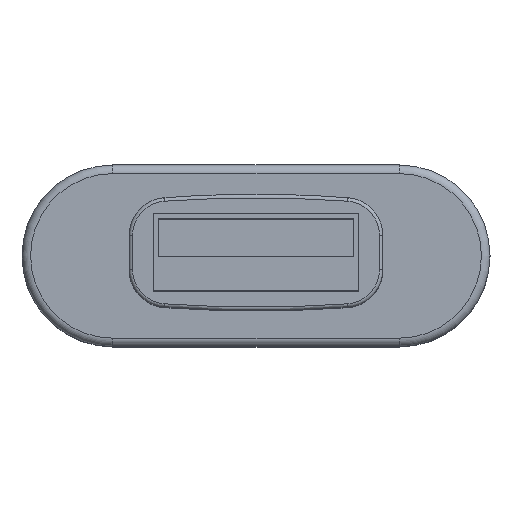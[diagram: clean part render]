
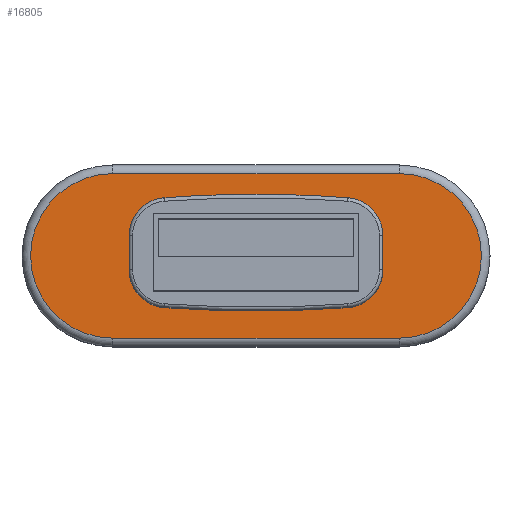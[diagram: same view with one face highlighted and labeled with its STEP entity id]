
A CAD part, top view. The second image highlights one B-rep face of the part: STEP entity #16805.
In plain terms, the highlighted planar face has unit normal (0, 0, 1).
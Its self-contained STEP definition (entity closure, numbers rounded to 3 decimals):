
#1 = EDGE_CURVE ( 'NONE', #7623, #8431, #138, .T. ) ;
#138 = LINE ( 'NONE', #15541, #14662 ) ;
#560 = CARTESIAN_POINT ( 'NONE',  ( -2.75, 0., 11.9 ) ) ;
#772 = CARTESIAN_POINT ( 'NONE',  ( 0., 0., 11.9 ) ) ;
#1634 = ORIENTED_EDGE ( 'NONE', *, *, #1, .T. ) ;
#2061 = AXIS2_PLACEMENT_3D ( 'NONE', #13892, #9554, #3925 ) ;
#2501 = EDGE_CURVE ( 'NONE', #7623, #11617, #17993, .T. ) ;
#2506 = FACE_OUTER_BOUND ( 'NONE', #5510, .T. ) ;
#2599 = DIRECTION ( 'NONE',  ( 1., 0., 0. ) ) ;
#2893 = EDGE_CURVE ( 'NONE', #12630, #16868, #10523, .T. ) ;
#2943 = ORIENTED_EDGE ( 'NONE', *, *, #2501, .F. ) ;
#3143 = EDGE_CURVE ( 'NONE', #16868, #12630, #8748, .T. ) ;
#3645 = CIRCLE ( 'NONE', #12779, 4.8 ) ;
#3925 = DIRECTION ( 'NONE',  ( 0.015, 1., 0. ) ) ;
#3985 = CARTESIAN_POINT ( 'NONE',  ( 0., 0., 11.9 ) ) ;
#4636 = AXIS2_PLACEMENT_3D ( 'NONE', #3985, #16712, #2599 ) ;
#5018 = EDGE_CURVE ( 'NONE', #6228, #8431, #3645, .T. ) ;
#5089 = VECTOR ( 'NONE', #16132, 1000. ) ;
#5510 = EDGE_LOOP ( 'NONE', ( #9092, #2943, #1634, #7938 ) ) ;
#5530 = CARTESIAN_POINT ( 'NONE',  ( -8.35, -4.8, 11.9 ) ) ;
#6102 = ORIENTED_EDGE ( 'NONE', *, *, #2893, .F. ) ;
#6228 = VERTEX_POINT ( 'NONE', #14705 ) ;
#6397 = AXIS2_PLACEMENT_3D ( 'NONE', #772, #10829, #12128 ) ;
#7404 = DIRECTION ( 'NONE',  ( -1., 0., 0. ) ) ;
#7623 = VERTEX_POINT ( 'NONE', #8288 ) ;
#7847 = EDGE_CURVE ( 'NONE', #6228, #11617, #12918, .T. ) ;
#7938 = ORIENTED_EDGE ( 'NONE', *, *, #5018, .F. ) ;
#8040 = CARTESIAN_POINT ( 'NONE',  ( -8.35, 4.8, 11.9 ) ) ;
#8288 = CARTESIAN_POINT ( 'NONE',  ( 8.35, 4.8, 11.9 ) ) ;
#8431 = VERTEX_POINT ( 'NONE', #8040 ) ;
#8748 = CIRCLE ( 'NONE', #11114, 2.75 ) ;
#9092 = ORIENTED_EDGE ( 'NONE', *, *, #7847, .T. ) ;
#9554 = DIRECTION ( 'NONE',  ( 0., 0., -1. ) ) ;
#9662 = CARTESIAN_POINT ( 'NONE',  ( 2.75, 0., 11.9 ) ) ;
#10480 = EDGE_LOOP ( 'NONE', ( #6102, #17722 ) ) ;
#10523 = CIRCLE ( 'NONE', #6397, 2.75 ) ;
#10829 = DIRECTION ( 'NONE',  ( 0., 0., 1. ) ) ;
#11114 = AXIS2_PLACEMENT_3D ( 'NONE', #16158, #16063, #15879 ) ;
#11220 = CARTESIAN_POINT ( 'NONE',  ( 8.35, -4.8, 11.9 ) ) ;
#11617 = VERTEX_POINT ( 'NONE', #11220 ) ;
#12128 = DIRECTION ( 'NONE',  ( -1., 0.022, 0. ) ) ;
#12630 = VERTEX_POINT ( 'NONE', #9662 ) ;
#12779 = AXIS2_PLACEMENT_3D ( 'NONE', #14356, #13430, #17296 ) ;
#12918 = LINE ( 'NONE', #5530, #5089 ) ;
#13430 = DIRECTION ( 'NONE',  ( 0., 0., -1. ) ) ;
#13892 = CARTESIAN_POINT ( 'NONE',  ( 8.35, 0., 11.9 ) ) ;
#14039 = PLANE ( 'NONE',  #4636 ) ;
#14356 = CARTESIAN_POINT ( 'NONE',  ( -8.35, 0., 11.9 ) ) ;
#14662 = VECTOR ( 'NONE', #7404, 1000. ) ;
#14705 = CARTESIAN_POINT ( 'NONE',  ( -8.35, -4.8, 11.9 ) ) ;
#15541 = CARTESIAN_POINT ( 'NONE',  ( 8.35, 4.8, 11.9 ) ) ;
#15879 = DIRECTION ( 'NONE',  ( 1., -0.022, 0. ) ) ;
#16063 = DIRECTION ( 'NONE',  ( 0., 0., 1. ) ) ;
#16132 = DIRECTION ( 'NONE',  ( 1., 0., 0. ) ) ;
#16158 = CARTESIAN_POINT ( 'NONE',  ( 0., 0., 11.9 ) ) ;
#16712 = DIRECTION ( 'NONE',  ( 0., 0., 1. ) ) ;
#16805 = ADVANCED_FACE ( 'NONE', ( #2506, #18108 ), #14039, .T. ) ;
#16868 = VERTEX_POINT ( 'NONE', #560 ) ;
#17296 = DIRECTION ( 'NONE',  ( -0.015, -1., 0. ) ) ;
#17722 = ORIENTED_EDGE ( 'NONE', *, *, #3143, .F. ) ;
#17993 = CIRCLE ( 'NONE', #2061, 4.8 ) ;
#18108 = FACE_BOUND ( 'NONE', #10480, .T. ) ;
